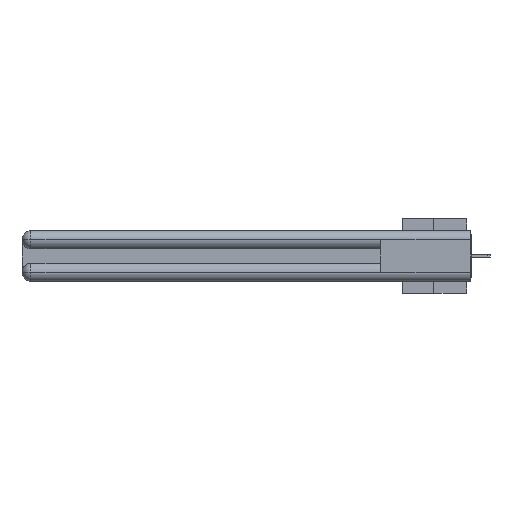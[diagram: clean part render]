
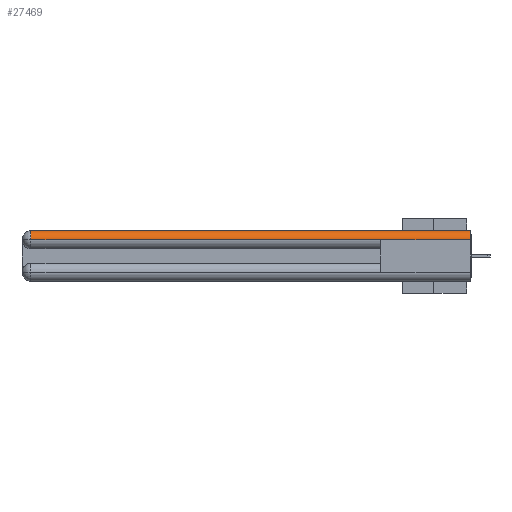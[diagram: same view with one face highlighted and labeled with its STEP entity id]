
A CAD part, left-side view. The second image highlights one B-rep face of the part: STEP entity #27469.
In plain terms, the highlighted cylindrical face has radius 1.562 mm (diameter 3.124 mm), a partial arc.
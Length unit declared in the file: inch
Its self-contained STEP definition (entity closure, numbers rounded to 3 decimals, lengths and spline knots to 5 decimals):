
#168 = AXIS2_PLACEMENT_3D ( 'NONE', #25855, #3013, #23547 ) ;
#627 = EDGE_CURVE ( 'NONE', #1572, #3937, #1151, .T. ) ;
#679 = ORIENTED_EDGE ( 'NONE', *, *, #13140, .F. ) ;
#754 = EDGE_LOOP ( 'NONE', ( #24139, #27640, #31074, #679, #15951 ) ) ;
#893 = DIRECTION ( 'NONE',  ( 0., 0., 1. ) ) ;
#1151 = LINE ( 'NONE', #8634, #30540 ) ;
#1311 = CARTESIAN_POINT ( 'NONE',  ( 0., 3., -0.0615 ) ) ;
#1497 = CARTESIAN_POINT ( 'NONE',  ( 0., 0., -0.0615 ) ) ;
#1572 = VERTEX_POINT ( 'NONE', #11678 ) ;
#2342 = DIRECTION ( 'NONE',  ( 1., 0., 0. ) ) ;
#2418 = VERTEX_POINT ( 'NONE', #5928 ) ;
#3013 = DIRECTION ( 'NONE',  ( 0., -1., 0. ) ) ;
#3937 = VERTEX_POINT ( 'NONE', #17774 ) ;
#4432 = CARTESIAN_POINT ( 'NONE',  ( 0., 0.6, -0.0615 ) ) ;
#4518 = CARTESIAN_POINT ( 'NONE',  ( 0.0615, 0., -0.0615 ) ) ;
#5928 = CARTESIAN_POINT ( 'NONE',  ( 0., 2.94, -0.0615 ) ) ;
#6206 = CARTESIAN_POINT ( 'NONE',  ( 0.0615, 0., -0.0615 ) ) ;
#6419 = EDGE_CURVE ( 'NONE', #2418, #13828, #23897, .T. ) ;
#7887 = EDGE_CURVE ( 'NONE', #3937, #9443, #7944, .T. ) ;
#7944 = CIRCLE ( 'NONE', #29742, 0.0615 ) ;
#8634 = CARTESIAN_POINT ( 'NONE',  ( 0.0615, 0., 0. ) ) ;
#9443 = VERTEX_POINT ( 'NONE', #1497 ) ;
#11639 = DIRECTION ( 'NONE',  ( 0., -1., 0. ) ) ;
#11678 = CARTESIAN_POINT ( 'NONE',  ( 0.0615, 2.94, 0. ) ) ;
#11806 = AXIS2_PLACEMENT_3D ( 'NONE', #6206, #26553, #893 ) ;
#13140 = EDGE_CURVE ( 'NONE', #9443, #13828, #29118, .T. ) ;
#13828 = VERTEX_POINT ( 'NONE', #4432 ) ;
#14362 = DIRECTION ( 'NONE',  ( 0., -1., 0. ) ) ;
#14552 = CIRCLE ( 'NONE', #168, 0.0615 ) ;
#15951 = ORIENTED_EDGE ( 'NONE', *, *, #7887, .F. ) ;
#17774 = CARTESIAN_POINT ( 'NONE',  ( 0.0615, 0., 0. ) ) ;
#18276 = VECTOR ( 'NONE', #21841, 39.37008 ) ;
#18744 = FACE_OUTER_BOUND ( 'NONE', #754, .T. ) ;
#21841 = DIRECTION ( 'NONE',  ( 0., 1., 0. ) ) ;
#22799 = VECTOR ( 'NONE', #31847, 39.37008 ) ;
#23547 = DIRECTION ( 'NONE',  ( 0., 0., 1. ) ) ;
#23897 = LINE ( 'NONE', #26694, #22799 ) ;
#24139 = ORIENTED_EDGE ( 'NONE', *, *, #627, .F. ) ;
#25855 = CARTESIAN_POINT ( 'NONE',  ( 0.0615, 2.94, -0.0615 ) ) ;
#26553 = DIRECTION ( 'NONE',  ( 0., 1., 0. ) ) ;
#26694 = CARTESIAN_POINT ( 'NONE',  ( 0., 3., -0.0615 ) ) ;
#26702 = EDGE_CURVE ( 'NONE', #1572, #2418, #14552, .T. ) ;
#27469 = ADVANCED_FACE ( 'NONE', ( #18744 ), #29029, .T. ) ;
#27640 = ORIENTED_EDGE ( 'NONE', *, *, #26702, .T. ) ;
#29029 = CYLINDRICAL_SURFACE ( 'NONE', #11806, 0.0615 ) ;
#29118 = LINE ( 'NONE', #1311, #18276 ) ;
#29742 = AXIS2_PLACEMENT_3D ( 'NONE', #4518, #14362, #2342 ) ;
#30540 = VECTOR ( 'NONE', #11639, 39.37008 ) ;
#31074 = ORIENTED_EDGE ( 'NONE', *, *, #6419, .T. ) ;
#31847 = DIRECTION ( 'NONE',  ( 0., -1., 0. ) ) ;
